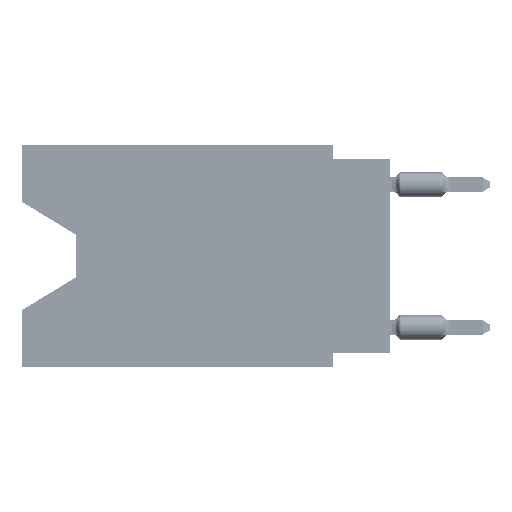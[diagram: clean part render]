
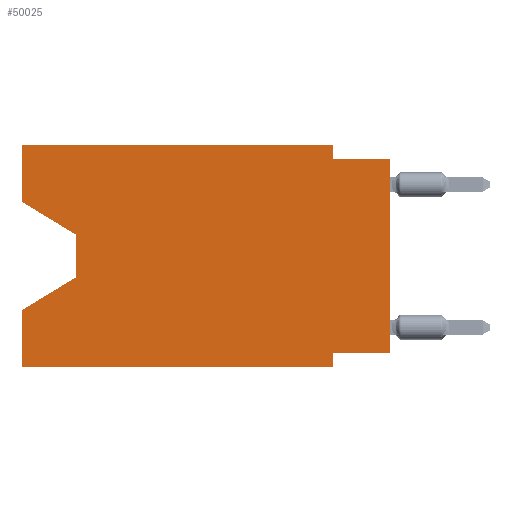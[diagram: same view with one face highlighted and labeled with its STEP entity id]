
A CAD part, left-side view. The second image highlights one B-rep face of the part: STEP entity #50025.
In plain terms, the highlighted planar face has unit normal (-1, 0, 0).
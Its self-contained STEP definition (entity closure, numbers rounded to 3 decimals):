
#221 = DIRECTION ( 'NONE',  ( 0., 0., 1. ) ) ;
#657 = DIRECTION ( 'NONE',  ( 0., 0., -1. ) ) ;
#1812 = CARTESIAN_POINT ( 'NONE',  ( 0., 2.54, -9.906 ) ) ;
#4397 = CARTESIAN_POINT ( 'NONE',  ( 0., 2.54, -0.635 ) ) ;
#4437 = VECTOR ( 'NONE', #657, 1000. ) ;
#4519 = EDGE_CURVE ( 'NONE', #14721, #14496, #71296, .T. ) ;
#5259 = CARTESIAN_POINT ( 'NONE',  ( 0., 16.383, 0. ) ) ;
#5740 = PLANE ( 'NONE',  #56456 ) ;
#5836 = CARTESIAN_POINT ( 'NONE',  ( 0., 2.54, 0. ) ) ;
#6123 = ORIENTED_EDGE ( 'NONE', *, *, #68617, .F. ) ;
#6169 = CARTESIAN_POINT ( 'NONE',  ( 0., 13.97, -5.893 ) ) ;
#6404 = DIRECTION ( 'NONE',  ( 0., 0., 1. ) ) ;
#7325 = LINE ( 'NONE', #26025, #70647 ) ;
#7704 = DIRECTION ( 'NONE',  ( 0., -1., 0. ) ) ;
#9184 = LINE ( 'NONE', #68620, #34491 ) ;
#9430 = EDGE_LOOP ( 'NONE', ( #70875, #52156, #28400, #71732, #19124, #6123, #48294, #59226, #24763, #16002, #16024, #30595 ) ) ;
#12838 = CARTESIAN_POINT ( 'NONE',  ( 0., 16.383, -7.36 ) ) ;
#13071 = CARTESIAN_POINT ( 'NONE',  ( 0., 13.97, -4.013 ) ) ;
#13225 = VECTOR ( 'NONE', #60302, 1000. ) ;
#14143 = LINE ( 'NONE', #39283, #72965 ) ;
#14496 = VERTEX_POINT ( 'NONE', #4397 ) ;
#14721 = VERTEX_POINT ( 'NONE', #49803 ) ;
#16002 = ORIENTED_EDGE ( 'NONE', *, *, #4519, .F. ) ;
#16024 = ORIENTED_EDGE ( 'NONE', *, *, #26460, .F. ) ;
#17562 = VERTEX_POINT ( 'NONE', #54994 ) ;
#18132 = VERTEX_POINT ( 'NONE', #51672 ) ;
#19124 = ORIENTED_EDGE ( 'NONE', *, *, #75593, .T. ) ;
#19878 = CARTESIAN_POINT ( 'NONE',  ( 0., 0., -0.635 ) ) ;
#20307 = VERTEX_POINT ( 'NONE', #51866 ) ;
#22619 = VECTOR ( 'NONE', #25648, 1000. ) ;
#23401 = EDGE_CURVE ( 'NONE', #48629, #58513, #43725, .T. ) ;
#23862 = VECTOR ( 'NONE', #73049, 1000. ) ;
#24418 = VECTOR ( 'NONE', #6404, 1000. ) ;
#24763 = ORIENTED_EDGE ( 'NONE', *, *, #51473, .F. ) ;
#25648 = DIRECTION ( 'NONE',  ( 0., 1., 0. ) ) ;
#26025 = CARTESIAN_POINT ( 'NONE',  ( 0., 0., -0.635 ) ) ;
#26460 = EDGE_CURVE ( 'NONE', #34758, #14721, #9184, .T. ) ;
#28400 = ORIENTED_EDGE ( 'NONE', *, *, #44186, .T. ) ;
#28565 = CARTESIAN_POINT ( 'NONE',  ( 0., 16.383, 0. ) ) ;
#29720 = DIRECTION ( 'NONE',  ( 0., 0.855, -0.519 ) ) ;
#30595 = ORIENTED_EDGE ( 'NONE', *, *, #40519, .F. ) ;
#31264 = LINE ( 'NONE', #68739, #22619 ) ;
#32172 = VECTOR ( 'NONE', #29720, 1000. ) ;
#34491 = VECTOR ( 'NONE', #39109, 1000. ) ;
#34758 = VERTEX_POINT ( 'NONE', #28565 ) ;
#35717 = LINE ( 'NONE', #60060, #32172 ) ;
#36451 = CARTESIAN_POINT ( 'NONE',  ( 0., 16.383, 0. ) ) ;
#36719 = LINE ( 'NONE', #67031, #24418 ) ;
#39109 = DIRECTION ( 'NONE',  ( 0., -1., 0. ) ) ;
#39283 = CARTESIAN_POINT ( 'NONE',  ( 0., 16.383, -2.546 ) ) ;
#39763 = VECTOR ( 'NONE', #40981, 1000. ) ;
#40519 = EDGE_CURVE ( 'NONE', #20307, #34758, #72830, .T. ) ;
#40981 = DIRECTION ( 'NONE',  ( 0., 0., -1. ) ) ;
#41978 = LINE ( 'NONE', #48714, #23862 ) ;
#42009 = CARTESIAN_POINT ( 'NONE',  ( 0., 16.383, -9.906 ) ) ;
#42917 = CARTESIAN_POINT ( 'NONE',  ( 0., 16.383, 0. ) ) ;
#43229 = EDGE_CURVE ( 'NONE', #18132, #70846, #36719, .T. ) ;
#43725 = LINE ( 'NONE', #74436, #4437 ) ;
#44186 = EDGE_CURVE ( 'NONE', #58513, #74463, #35717, .T. ) ;
#47246 = FACE_OUTER_BOUND ( 'NONE', #9430, .T. ) ;
#48294 = ORIENTED_EDGE ( 'NONE', *, *, #68385, .F. ) ;
#48629 = VERTEX_POINT ( 'NONE', #13071 ) ;
#48714 = CARTESIAN_POINT ( 'NONE',  ( 0., 2.54, -9.906 ) ) ;
#49803 = CARTESIAN_POINT ( 'NONE',  ( 0., 2.54, 0. ) ) ;
#50025 = ADVANCED_FACE ( 'NONE', ( #47246 ), #5740, .F. ) ;
#50397 = EDGE_CURVE ( 'NONE', #51497, #74463, #54325, .T. ) ;
#50991 = VERTEX_POINT ( 'NONE', #1812 ) ;
#51473 = EDGE_CURVE ( 'NONE', #14496, #70846, #7325, .T. ) ;
#51497 = VERTEX_POINT ( 'NONE', #52769 ) ;
#51672 = CARTESIAN_POINT ( 'NONE',  ( 0., 0., -9.271 ) ) ;
#51866 = CARTESIAN_POINT ( 'NONE',  ( 0., 16.383, -2.546 ) ) ;
#52156 = ORIENTED_EDGE ( 'NONE', *, *, #23401, .T. ) ;
#52769 = CARTESIAN_POINT ( 'NONE',  ( 0., 16.383, -9.906 ) ) ;
#54325 = LINE ( 'NONE', #5259, #13225 ) ;
#54994 = CARTESIAN_POINT ( 'NONE',  ( 0., 2.54, -9.271 ) ) ;
#56456 = AXIS2_PLACEMENT_3D ( 'NONE', #36451, #71973, #60799 ) ;
#56458 = EDGE_CURVE ( 'NONE', #20307, #48629, #14143, .T. ) ;
#58513 = VERTEX_POINT ( 'NONE', #6169 ) ;
#59226 = ORIENTED_EDGE ( 'NONE', *, *, #43229, .T. ) ;
#60060 = CARTESIAN_POINT ( 'NONE',  ( 0., 13.97, -5.893 ) ) ;
#60302 = DIRECTION ( 'NONE',  ( 0., 0., 1. ) ) ;
#60799 = DIRECTION ( 'NONE',  ( 0., 0., -1. ) ) ;
#63624 = DIRECTION ( 'NONE',  ( 0., -0.855, -0.519 ) ) ;
#65550 = LINE ( 'NONE', #42009, #70979 ) ;
#67031 = CARTESIAN_POINT ( 'NONE',  ( 0., 0., 0. ) ) ;
#68385 = EDGE_CURVE ( 'NONE', #18132, #17562, #31264, .T. ) ;
#68617 = EDGE_CURVE ( 'NONE', #17562, #50991, #41978, .T. ) ;
#68620 = CARTESIAN_POINT ( 'NONE',  ( 0., 16.383, 0. ) ) ;
#68739 = CARTESIAN_POINT ( 'NONE',  ( 0., 0., -9.271 ) ) ;
#70647 = VECTOR ( 'NONE', #7704, 1000. ) ;
#70846 = VERTEX_POINT ( 'NONE', #19878 ) ;
#70875 = ORIENTED_EDGE ( 'NONE', *, *, #56458, .T. ) ;
#70979 = VECTOR ( 'NONE', #71542, 1000. ) ;
#71296 = LINE ( 'NONE', #5836, #39763 ) ;
#71542 = DIRECTION ( 'NONE',  ( 0., -1., 0. ) ) ;
#71732 = ORIENTED_EDGE ( 'NONE', *, *, #50397, .F. ) ;
#71973 = DIRECTION ( 'NONE',  ( 1., 0., 0. ) ) ;
#72303 = VECTOR ( 'NONE', #221, 1000. ) ;
#72830 = LINE ( 'NONE', #42917, #72303 ) ;
#72965 = VECTOR ( 'NONE', #63624, 1000. ) ;
#73049 = DIRECTION ( 'NONE',  ( 0., 0., -1. ) ) ;
#74436 = CARTESIAN_POINT ( 'NONE',  ( 0., 13.97, -4.013 ) ) ;
#74463 = VERTEX_POINT ( 'NONE', #12838 ) ;
#75593 = EDGE_CURVE ( 'NONE', #51497, #50991, #65550, .T. ) ;
